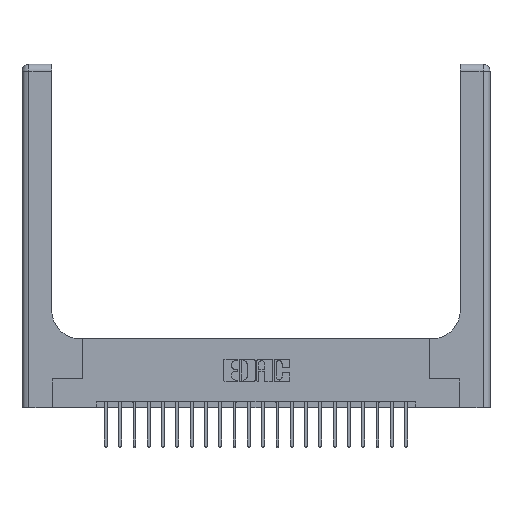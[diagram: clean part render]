
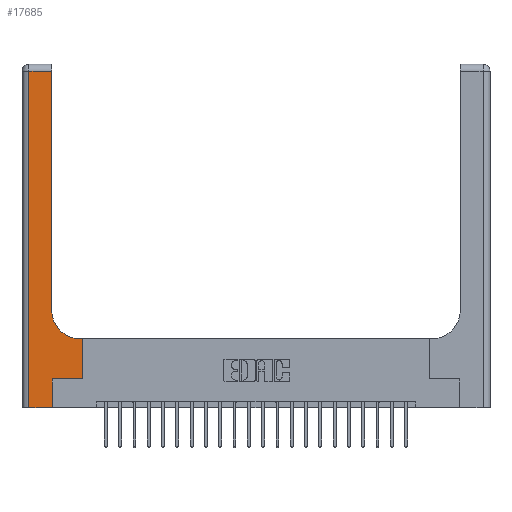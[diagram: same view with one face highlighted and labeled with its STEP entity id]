
A CAD part, top view. The second image highlights one B-rep face of the part: STEP entity #17685.
In plain terms, the highlighted planar face has unit normal (0, 0, 1).
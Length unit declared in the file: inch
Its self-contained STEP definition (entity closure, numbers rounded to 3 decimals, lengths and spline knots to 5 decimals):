
#325 = VECTOR ( 'NONE', #2766, 39.37008 ) ;
#416 = VERTEX_POINT ( 'NONE', #13550 ) ;
#445 = ORIENTED_EDGE ( 'NONE', *, *, #18718, .T. ) ;
#493 = DIRECTION ( 'NONE',  ( -1., 0., 0. ) ) ;
#669 = LINE ( 'NONE', #2391, #16693 ) ;
#908 = CARTESIAN_POINT ( 'NONE',  ( 0.06, 2.94, 0.37 ) ) ;
#1081 = CARTESIAN_POINT ( 'NONE',  ( 0.265, 0.25, 0.37 ) ) ;
#1129 = EDGE_CURVE ( 'NONE', #10671, #17451, #9133, .T. ) ;
#1143 = DIRECTION ( 'NONE',  ( 1., 0., 0. ) ) ;
#1146 = CARTESIAN_POINT ( 'NONE',  ( 0.06, 0., 0.37 ) ) ;
#1735 = ORIENTED_EDGE ( 'NONE', *, *, #1129, .T. ) ;
#2034 = DIRECTION ( 'NONE',  ( 0., 0., -1. ) ) ;
#2391 = CARTESIAN_POINT ( 'NONE',  ( 0.265, 0.25, 0.37 ) ) ;
#2741 = CARTESIAN_POINT ( 'NONE',  ( 0., 0., 0.37 ) ) ;
#2766 = DIRECTION ( 'NONE',  ( 0., 1., 0. ) ) ;
#2945 = VERTEX_POINT ( 'NONE', #22042 ) ;
#3870 = DIRECTION ( 'NONE',  ( 1., 0., 0. ) ) ;
#3962 = PLANE ( 'NONE',  #7015 ) ;
#4005 = LINE ( 'NONE', #10925, #13937 ) ;
#4113 = CARTESIAN_POINT ( 'NONE',  ( 0.26, 2.94, 0.37 ) ) ;
#4368 = LINE ( 'NONE', #7985, #9507 ) ;
#5257 = CIRCLE ( 'NONE', #13633, 0.25 ) ;
#6074 = DIRECTION ( 'NONE',  ( 0., -1., 0. ) ) ;
#6154 = CARTESIAN_POINT ( 'NONE',  ( 0.265, 0., 0.37 ) ) ;
#7015 = AXIS2_PLACEMENT_3D ( 'NONE', #14131, #2034, #8952 ) ;
#7417 = ORIENTED_EDGE ( 'NONE', *, *, #8852, .T. ) ;
#7985 = CARTESIAN_POINT ( 'NONE',  ( 0.06, 3., 0.37 ) ) ;
#8773 = DIRECTION ( 'NONE',  ( 0., 1., 0. ) ) ;
#8852 = EDGE_CURVE ( 'NONE', #416, #10671, #11510, .T. ) ;
#8952 = DIRECTION ( 'NONE',  ( -1., 0., 0. ) ) ;
#9133 = LINE ( 'NONE', #16173, #20433 ) ;
#9507 = VECTOR ( 'NONE', #6074, 39.37008 ) ;
#9714 = ORIENTED_EDGE ( 'NONE', *, *, #11918, .T. ) ;
#9743 = CARTESIAN_POINT ( 'NONE',  ( 0.265, 0., 0.37 ) ) ;
#10671 = VERTEX_POINT ( 'NONE', #4113 ) ;
#10683 = EDGE_CURVE ( 'NONE', #21722, #22178, #18230, .T. ) ;
#10925 = CARTESIAN_POINT ( 'NONE',  ( 0.528, 0.25, 0.37 ) ) ;
#11025 = LINE ( 'NONE', #19065, #15119 ) ;
#11510 = LINE ( 'NONE', #14984, #325 ) ;
#11787 = CARTESIAN_POINT ( 'NONE',  ( 0.528, 0.25, 0.37 ) ) ;
#11918 = EDGE_CURVE ( 'NONE', #22695, #22581, #4005, .T. ) ;
#12304 = DIRECTION ( 'NONE',  ( 0., 0., -1. ) ) ;
#12482 = VECTOR ( 'NONE', #13126, 39.37008 ) ;
#12603 = EDGE_CURVE ( 'NONE', #22581, #2945, #11025, .T. ) ;
#13126 = DIRECTION ( 'NONE',  ( 0., 1., 0. ) ) ;
#13550 = CARTESIAN_POINT ( 'NONE',  ( 0.26, 0.85, 0.37 ) ) ;
#13633 = AXIS2_PLACEMENT_3D ( 'NONE', #19234, #12304, #15877 ) ;
#13772 = ORIENTED_EDGE ( 'NONE', *, *, #15165, .T. ) ;
#13937 = VECTOR ( 'NONE', #8773, 39.37008 ) ;
#14131 = CARTESIAN_POINT ( 'NONE',  ( 0., 3., 0.37 ) ) ;
#14242 = ORIENTED_EDGE ( 'NONE', *, *, #15634, .T. ) ;
#14984 = CARTESIAN_POINT ( 'NONE',  ( 0.26, 3., 0.37 ) ) ;
#15119 = VECTOR ( 'NONE', #18114, 39.37008 ) ;
#15165 = EDGE_CURVE ( 'NONE', #17451, #21722, #4368, .T. ) ;
#15634 = EDGE_CURVE ( 'NONE', #22178, #18202, #18120, .T. ) ;
#15877 = DIRECTION ( 'NONE',  ( 1., 0., 0. ) ) ;
#16173 = CARTESIAN_POINT ( 'NONE',  ( 0., 2.94, 0.37 ) ) ;
#16214 = FACE_OUTER_BOUND ( 'NONE', #21423, .T. ) ;
#16647 = ORIENTED_EDGE ( 'NONE', *, *, #12603, .T. ) ;
#16693 = VECTOR ( 'NONE', #3870, 39.37008 ) ;
#16986 = ORIENTED_EDGE ( 'NONE', *, *, #10683, .T. ) ;
#17451 = VERTEX_POINT ( 'NONE', #908 ) ;
#17685 = ADVANCED_FACE ( 'NONE', ( #16214 ), #3962, .F. ) ;
#18114 = DIRECTION ( 'NONE',  ( -1., 0., 0. ) ) ;
#18120 = LINE ( 'NONE', #6154, #12482 ) ;
#18202 = VERTEX_POINT ( 'NONE', #1081 ) ;
#18230 = LINE ( 'NONE', #2741, #20815 ) ;
#18718 = EDGE_CURVE ( 'NONE', #2945, #416, #5257, .T. ) ;
#19065 = CARTESIAN_POINT ( 'NONE',  ( 0.26, 0.6, 0.37 ) ) ;
#19234 = CARTESIAN_POINT ( 'NONE',  ( 0.51, 0.85, 0.37 ) ) ;
#20433 = VECTOR ( 'NONE', #493, 39.37008 ) ;
#20660 = ORIENTED_EDGE ( 'NONE', *, *, #21960, .T. ) ;
#20815 = VECTOR ( 'NONE', #1143, 39.37008 ) ;
#21423 = EDGE_LOOP ( 'NONE', ( #7417, #1735, #13772, #16986, #14242, #20660, #9714, #16647, #445 ) ) ;
#21722 = VERTEX_POINT ( 'NONE', #1146 ) ;
#21868 = CARTESIAN_POINT ( 'NONE',  ( 0.528, 0.6, 0.37 ) ) ;
#21960 = EDGE_CURVE ( 'NONE', #18202, #22695, #669, .T. ) ;
#22042 = CARTESIAN_POINT ( 'NONE',  ( 0.51, 0.6, 0.37 ) ) ;
#22178 = VERTEX_POINT ( 'NONE', #9743 ) ;
#22581 = VERTEX_POINT ( 'NONE', #21868 ) ;
#22695 = VERTEX_POINT ( 'NONE', #11787 ) ;
